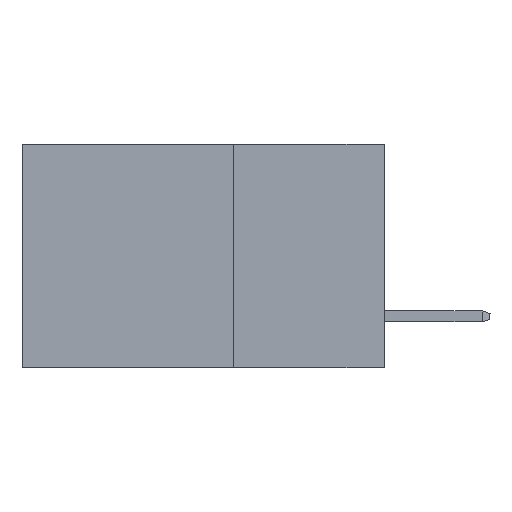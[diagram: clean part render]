
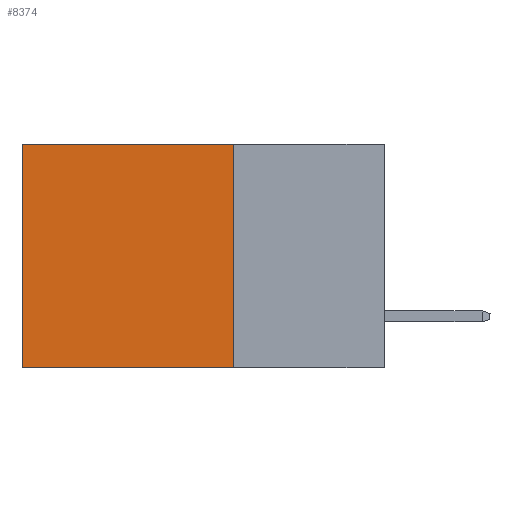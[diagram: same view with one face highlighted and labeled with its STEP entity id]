
A CAD part, left-side view. The second image highlights one B-rep face of the part: STEP entity #8374.
In plain terms, the highlighted planar face has unit normal (-1, 0, 0).
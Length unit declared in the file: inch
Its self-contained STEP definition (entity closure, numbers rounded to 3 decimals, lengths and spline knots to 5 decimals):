
#559 = DIRECTION ( 'NONE',  ( 0., 0., -1. ) ) ;
#1151 = VERTEX_POINT ( 'NONE', #5779 ) ;
#1499 = CARTESIAN_POINT ( 'NONE',  ( 0.2615, 0.25, -0.37 ) ) ;
#2605 = LINE ( 'NONE', #1499, #7462 ) ;
#3102 = AXIS2_PLACEMENT_3D ( 'NONE', #3923, #8386, #559 ) ;
#3481 = LINE ( 'NONE', #5527, #4516 ) ;
#3923 = CARTESIAN_POINT ( 'NONE',  ( 0.2615, 0.25, -0.37 ) ) ;
#4512 = EDGE_CURVE ( 'NONE', #11958, #6510, #2605, .T. ) ;
#4516 = VECTOR ( 'NONE', #6846, 39.37008 ) ;
#5007 = DIRECTION ( 'NONE',  ( 0., 0., -1. ) ) ;
#5297 = DIRECTION ( 'NONE',  ( 0., 0., -1. ) ) ;
#5496 = EDGE_LOOP ( 'NONE', ( #12857, #11628, #13420, #11672 ) ) ;
#5527 = CARTESIAN_POINT ( 'NONE',  ( 0.2615, 0.25, 0. ) ) ;
#5547 = CARTESIAN_POINT ( 'NONE',  ( 0.2615, 0.6, -0.37 ) ) ;
#5779 = CARTESIAN_POINT ( 'NONE',  ( 0.2615, 0.6, -0.37 ) ) ;
#6403 = CARTESIAN_POINT ( 'NONE',  ( 0.2615, 0.6, 0. ) ) ;
#6510 = VERTEX_POINT ( 'NONE', #10954 ) ;
#6846 = DIRECTION ( 'NONE',  ( 0., 1., 0. ) ) ;
#7137 = PLANE ( 'NONE',  #3102 ) ;
#7462 = VECTOR ( 'NONE', #5007, 39.37008 ) ;
#8374 = ADVANCED_FACE ( 'NONE', ( #12826 ), #7137, .F. ) ;
#8386 = DIRECTION ( 'NONE',  ( 1., 0., 0. ) ) ;
#8536 = VERTEX_POINT ( 'NONE', #6403 ) ;
#8982 = EDGE_CURVE ( 'NONE', #6510, #1151, #14164, .T. ) ;
#9679 = EDGE_CURVE ( 'NONE', #8536, #1151, #12461, .T. ) ;
#9945 = EDGE_CURVE ( 'NONE', #11958, #8536, #3481, .T. ) ;
#10954 = CARTESIAN_POINT ( 'NONE',  ( 0.2615, 0.25, -0.37 ) ) ;
#11628 = ORIENTED_EDGE ( 'NONE', *, *, #8982, .F. ) ;
#11672 = ORIENTED_EDGE ( 'NONE', *, *, #9945, .T. ) ;
#11958 = VERTEX_POINT ( 'NONE', #12332 ) ;
#12332 = CARTESIAN_POINT ( 'NONE',  ( 0.2615, 0.25, 0. ) ) ;
#12461 = LINE ( 'NONE', #5547, #13591 ) ;
#12826 = FACE_OUTER_BOUND ( 'NONE', #5496, .T. ) ;
#12857 = ORIENTED_EDGE ( 'NONE', *, *, #9679, .T. ) ;
#13222 = DIRECTION ( 'NONE',  ( 0., 1., 0. ) ) ;
#13337 = VECTOR ( 'NONE', #13222, 39.37008 ) ;
#13420 = ORIENTED_EDGE ( 'NONE', *, *, #4512, .F. ) ;
#13591 = VECTOR ( 'NONE', #5297, 39.37008 ) ;
#14164 = LINE ( 'NONE', #14385, #13337 ) ;
#14385 = CARTESIAN_POINT ( 'NONE',  ( 0.2615, 0.25, -0.37 ) ) ;
